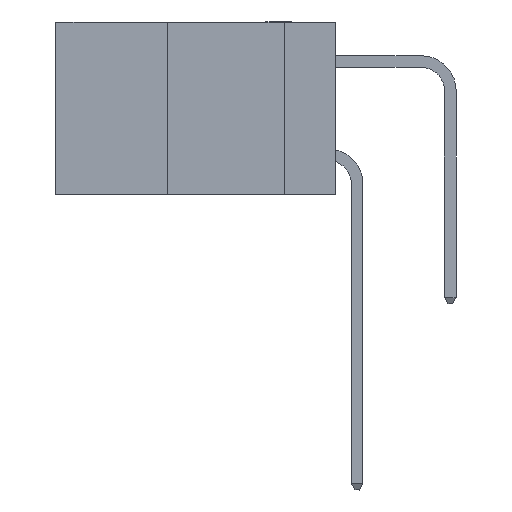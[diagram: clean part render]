
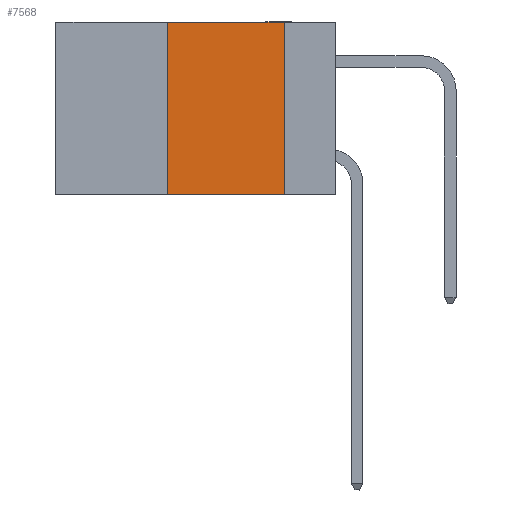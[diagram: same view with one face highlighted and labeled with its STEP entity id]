
A CAD part, left-side view. The second image highlights one B-rep face of the part: STEP entity #7568.
In plain terms, the highlighted planar face has unit normal (-1, 0, 0).
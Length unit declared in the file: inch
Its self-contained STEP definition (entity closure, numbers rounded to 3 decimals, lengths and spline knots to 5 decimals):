
#523 = FACE_OUTER_BOUND ( 'NONE', #20541, .T. ) ;
#1394 = EDGE_CURVE ( 'NONE', #4766, #2330, #9096, .T. ) ;
#1986 = PLANE ( 'NONE',  #2217 ) ;
#2203 = VECTOR ( 'NONE', #18956, 39.37008 ) ;
#2217 = AXIS2_PLACEMENT_3D ( 'NONE', #18069, #13221, #11529 ) ;
#2330 = VERTEX_POINT ( 'NONE', #16288 ) ;
#2405 = VECTOR ( 'NONE', #10414, 39.37008 ) ;
#4432 = CARTESIAN_POINT ( 'NONE',  ( 0., 0.36, 0. ) ) ;
#4766 = VERTEX_POINT ( 'NONE', #6277 ) ;
#5627 = EDGE_CURVE ( 'NONE', #17851, #2330, #12811, .T. ) ;
#5741 = ORIENTED_EDGE ( 'NONE', *, *, #1394, .T. ) ;
#5916 = CARTESIAN_POINT ( 'NONE',  ( 0., 0.6, -0.37 ) ) ;
#5986 = EDGE_CURVE ( 'NONE', #7769, #17851, #20195, .T. ) ;
#6277 = CARTESIAN_POINT ( 'NONE',  ( 0., 0.36, -0.37 ) ) ;
#6886 = EDGE_CURVE ( 'NONE', #4766, #7769, #17170, .T. ) ;
#6925 = ORIENTED_EDGE ( 'NONE', *, *, #5986, .F. ) ;
#7270 = VECTOR ( 'NONE', #17891, 39.37008 ) ;
#7568 = ADVANCED_FACE ( 'NONE', ( #523 ), #1986, .F. ) ;
#7769 = VERTEX_POINT ( 'NONE', #15338 ) ;
#9096 = LINE ( 'NONE', #5916, #2405 ) ;
#9414 = CARTESIAN_POINT ( 'NONE',  ( 0., 0.11, 0. ) ) ;
#10414 = DIRECTION ( 'NONE',  ( 0., -1., 0. ) ) ;
#10685 = DIRECTION ( 'NONE',  ( 0., -1., 0. ) ) ;
#11017 = ORIENTED_EDGE ( 'NONE', *, *, #5627, .F. ) ;
#11315 = VECTOR ( 'NONE', #10685, 39.37008 ) ;
#11529 = DIRECTION ( 'NONE',  ( 0., 0., -1. ) ) ;
#12811 = LINE ( 'NONE', #9414, #7270 ) ;
#13221 = DIRECTION ( 'NONE',  ( 1., 0., 0. ) ) ;
#15338 = CARTESIAN_POINT ( 'NONE',  ( 0., 0.36, 0. ) ) ;
#16288 = CARTESIAN_POINT ( 'NONE',  ( 0., 0.11, -0.37 ) ) ;
#17170 = LINE ( 'NONE', #4432, #2203 ) ;
#17263 = CARTESIAN_POINT ( 'NONE',  ( 0., 0.11, 0. ) ) ;
#17851 = VERTEX_POINT ( 'NONE', #17263 ) ;
#17891 = DIRECTION ( 'NONE',  ( 0., 0., -1. ) ) ;
#18069 = CARTESIAN_POINT ( 'NONE',  ( 0., 0.6, 0. ) ) ;
#18956 = DIRECTION ( 'NONE',  ( 0., 0., 1. ) ) ;
#19528 = ORIENTED_EDGE ( 'NONE', *, *, #6886, .F. ) ;
#20195 = LINE ( 'NONE', #20297, #11315 ) ;
#20297 = CARTESIAN_POINT ( 'NONE',  ( 0., 0.6, 0. ) ) ;
#20541 = EDGE_LOOP ( 'NONE', ( #11017, #6925, #19528, #5741 ) ) ;
